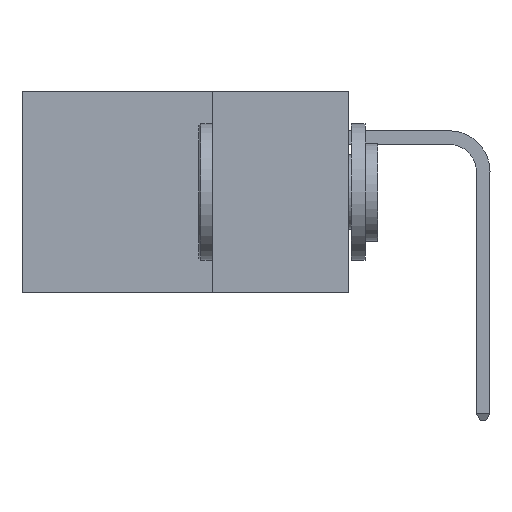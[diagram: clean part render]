
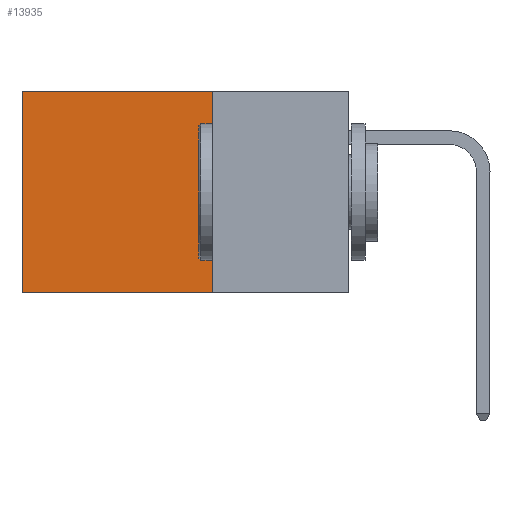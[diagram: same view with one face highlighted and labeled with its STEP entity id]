
A CAD part, left-side view. The second image highlights one B-rep face of the part: STEP entity #13935.
In plain terms, the highlighted planar face has unit normal (-1, 0, 0).
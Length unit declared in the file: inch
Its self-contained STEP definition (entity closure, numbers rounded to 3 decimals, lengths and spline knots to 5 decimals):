
#109 = VECTOR ( 'NONE', #13834, 39.37008 ) ;
#172 = ORIENTED_EDGE ( 'NONE', *, *, #15631, .F. ) ;
#205 = CARTESIAN_POINT ( 'NONE',  ( 0.2875, 0.25, -0.37 ) ) ;
#375 = LINE ( 'NONE', #1391, #4588 ) ;
#546 = LINE ( 'NONE', #8748, #18034 ) ;
#597 = LINE ( 'NONE', #5701, #4800 ) ;
#659 = CARTESIAN_POINT ( 'NONE',  ( 0.2875, 0.25, -0.37 ) ) ;
#1391 = CARTESIAN_POINT ( 'NONE',  ( 0.2875, 0.25, 0. ) ) ;
#1474 = DIRECTION ( 'NONE',  ( 0., 0., -1. ) ) ;
#3832 = EDGE_CURVE ( 'NONE', #6573, #21164, #546, .T. ) ;
#4382 = VERTEX_POINT ( 'NONE', #8523 ) ;
#4588 = VECTOR ( 'NONE', #1474, 39.37008 ) ;
#4800 = VECTOR ( 'NONE', #7495, 39.37008 ) ;
#5309 = VERTEX_POINT ( 'NONE', #659 ) ;
#5429 = LINE ( 'NONE', #205, #109 ) ;
#5478 = EDGE_LOOP ( 'NONE', ( #21410, #172, #18356, #16137 ) ) ;
#5701 = CARTESIAN_POINT ( 'NONE',  ( 0.2875, 0.25, 0. ) ) ;
#6573 = VERTEX_POINT ( 'NONE', #14129 ) ;
#7495 = DIRECTION ( 'NONE',  ( 0., 1., 0. ) ) ;
#8039 = EDGE_CURVE ( 'NONE', #4382, #5309, #375, .T. ) ;
#8523 = CARTESIAN_POINT ( 'NONE',  ( 0.2875, 0.25, 0. ) ) ;
#8626 = FACE_OUTER_BOUND ( 'NONE', #5478, .T. ) ;
#8748 = CARTESIAN_POINT ( 'NONE',  ( 0.2875, 0.6, 0. ) ) ;
#9627 = DIRECTION ( 'NONE',  ( 1., 0., 0. ) ) ;
#10418 = DIRECTION ( 'NONE',  ( 0., 0., -1. ) ) ;
#13834 = DIRECTION ( 'NONE',  ( 0., 1., 0. ) ) ;
#13935 = ADVANCED_FACE ( 'NONE', ( #8626 ), #19507, .F. ) ;
#14129 = CARTESIAN_POINT ( 'NONE',  ( 0.2875, 0.6, 0. ) ) ;
#14993 = AXIS2_PLACEMENT_3D ( 'NONE', #16213, #9627, #21149 ) ;
#15631 = EDGE_CURVE ( 'NONE', #5309, #21164, #5429, .T. ) ;
#16047 = CARTESIAN_POINT ( 'NONE',  ( 0.2875, 0.6, -0.37 ) ) ;
#16137 = ORIENTED_EDGE ( 'NONE', *, *, #18017, .T. ) ;
#16213 = CARTESIAN_POINT ( 'NONE',  ( 0.2875, 0.25, 0. ) ) ;
#18017 = EDGE_CURVE ( 'NONE', #4382, #6573, #597, .T. ) ;
#18034 = VECTOR ( 'NONE', #10418, 39.37008 ) ;
#18356 = ORIENTED_EDGE ( 'NONE', *, *, #8039, .F. ) ;
#19507 = PLANE ( 'NONE',  #14993 ) ;
#21149 = DIRECTION ( 'NONE',  ( 0., 0., -1. ) ) ;
#21164 = VERTEX_POINT ( 'NONE', #16047 ) ;
#21410 = ORIENTED_EDGE ( 'NONE', *, *, #3832, .T. ) ;
